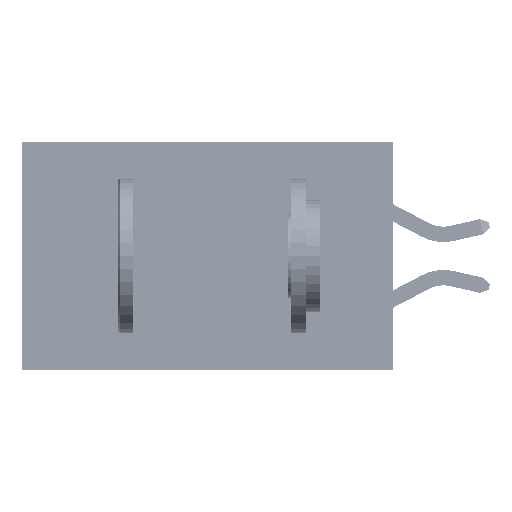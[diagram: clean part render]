
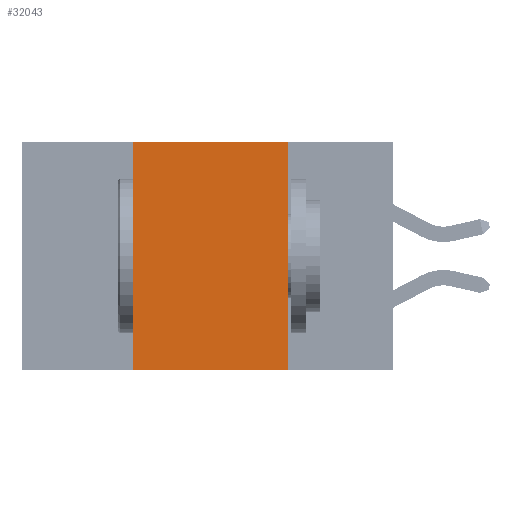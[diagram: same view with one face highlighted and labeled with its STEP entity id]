
A CAD part, left-side view. The second image highlights one B-rep face of the part: STEP entity #32043.
In plain terms, the highlighted planar face has unit normal (-1, 0, 0).
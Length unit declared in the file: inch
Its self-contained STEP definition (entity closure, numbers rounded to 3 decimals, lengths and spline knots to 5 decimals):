
#2175 = CARTESIAN_POINT ( 'NONE',  ( 0., 0.17, 0. ) ) ;
#3389 = VERTEX_POINT ( 'NONE', #42330 ) ;
#4764 = CARTESIAN_POINT ( 'NONE',  ( 0., 0.42, 0. ) ) ;
#6096 = CARTESIAN_POINT ( 'NONE',  ( 0., 0.6, 0. ) ) ;
#7086 = CARTESIAN_POINT ( 'NONE',  ( 0., 0.6, 0. ) ) ;
#11223 = CARTESIAN_POINT ( 'NONE',  ( 0., 0.6, -0.37 ) ) ;
#12701 = ORIENTED_EDGE ( 'NONE', *, *, #33198, .F. ) ;
#13391 = AXIS2_PLACEMENT_3D ( 'NONE', #6096, #47491, #25146 ) ;
#13620 = LINE ( 'NONE', #2175, #42385 ) ;
#14054 = CARTESIAN_POINT ( 'NONE',  ( 0., 0.42, -0.37 ) ) ;
#15439 = EDGE_CURVE ( 'NONE', #41917, #23018, #16092, .T. ) ;
#16092 = LINE ( 'NONE', #11223, #42468 ) ;
#16331 = VECTOR ( 'NONE', #44588, 39.37008 ) ;
#20011 = ORIENTED_EDGE ( 'NONE', *, *, #31321, .F. ) ;
#21356 = PLANE ( 'NONE',  #13391 ) ;
#21572 = ORIENTED_EDGE ( 'NONE', *, *, #47713, .F. ) ;
#21831 = FACE_OUTER_BOUND ( 'NONE', #47579, .T. ) ;
#23018 = VERTEX_POINT ( 'NONE', #33453 ) ;
#23914 = CARTESIAN_POINT ( 'NONE',  ( 0., 0.42, 0. ) ) ;
#25047 = DIRECTION ( 'NONE',  ( 0., 0., -1. ) ) ;
#25146 = DIRECTION ( 'NONE',  ( 0., 0., -1. ) ) ;
#29916 = LINE ( 'NONE', #23914, #47429 ) ;
#31321 = EDGE_CURVE ( 'NONE', #3389, #23018, #13620, .T. ) ;
#32043 = ADVANCED_FACE ( 'NONE', ( #21831 ), #21356, .F. ) ;
#33198 = EDGE_CURVE ( 'NONE', #41917, #42726, #29916, .T. ) ;
#33453 = CARTESIAN_POINT ( 'NONE',  ( 0., 0.17, -0.37 ) ) ;
#37444 = LINE ( 'NONE', #7086, #16331 ) ;
#37513 = DIRECTION ( 'NONE',  ( 0., -1., 0. ) ) ;
#38926 = DIRECTION ( 'NONE',  ( 0., 0., 1. ) ) ;
#41917 = VERTEX_POINT ( 'NONE', #14054 ) ;
#42330 = CARTESIAN_POINT ( 'NONE',  ( 0., 0.17, 0. ) ) ;
#42385 = VECTOR ( 'NONE', #25047, 39.37008 ) ;
#42468 = VECTOR ( 'NONE', #37513, 39.37008 ) ;
#42649 = ORIENTED_EDGE ( 'NONE', *, *, #15439, .T. ) ;
#42726 = VERTEX_POINT ( 'NONE', #4764 ) ;
#44588 = DIRECTION ( 'NONE',  ( 0., -1., 0. ) ) ;
#47429 = VECTOR ( 'NONE', #38926, 39.37008 ) ;
#47491 = DIRECTION ( 'NONE',  ( 1., 0., 0. ) ) ;
#47579 = EDGE_LOOP ( 'NONE', ( #20011, #21572, #12701, #42649 ) ) ;
#47713 = EDGE_CURVE ( 'NONE', #42726, #3389, #37444, .T. ) ;
